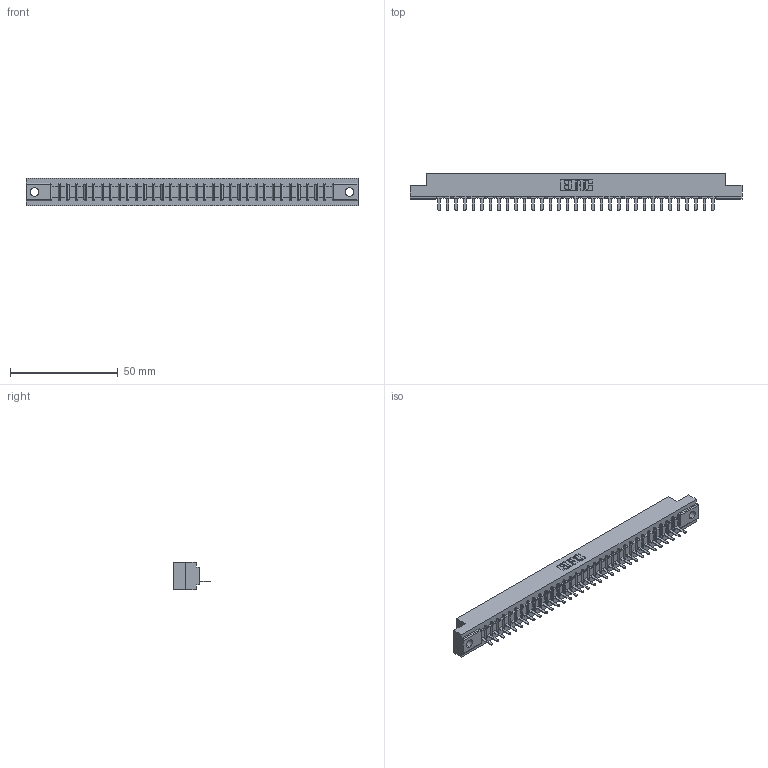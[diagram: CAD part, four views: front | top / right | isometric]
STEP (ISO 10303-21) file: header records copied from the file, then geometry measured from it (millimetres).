
FILE_DESCRIPTION (( 'STEP AP203' ), '1' );
FILE_NAME ('307-033-521-104.STEP', '2019-09-05T05:51:10', ( '' ), ( '' ), 'SwSTEP 2.0', 'SolidWorks 2016', '' );
FILE_SCHEMA (( 'CONFIG_CONTROL_DESIGN' ));
Length unit declared in the file: inch
Products named in the file (3): 307-290-002_521; 307-033-521-104; 307 Part_.156 Dia Mounting Holes
Assembly tree (34 placements, depth 2):
  307-033-521-104
    307 Part_.156 Dia Mounting Holes
    307-290-002_521  x33
Bounding box: 153.77 x 17.42 x 12.7 mm (x, y, z)
Volume: 16284.4 mm3; surface area: 20119.6 mm2
Topology: 34 solids, 34 shells, 2608 faces, 8015 edges, 5250 vertices
Faces by surface type: plane 1569, cylinder 971, sphere 68
Entity records: 30536 total; most frequent: CARTESIAN_POINT 5154, ORIENTED_EDGE 5142, DIRECTION 5003, EDGE_CURVE 2571, VECTOR 1973, LINE 1973, VERTEX_POINT 1666, AXIS2_PLACEMENT_3D 1515
